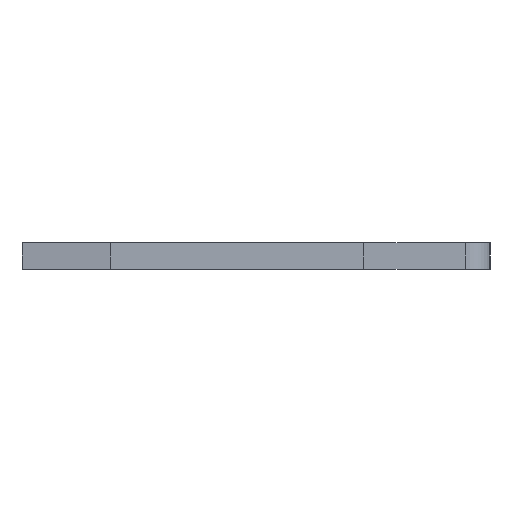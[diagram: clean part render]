
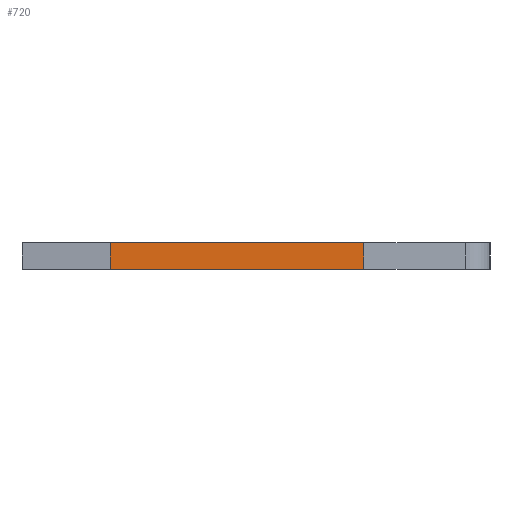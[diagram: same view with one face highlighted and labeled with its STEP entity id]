
A CAD part, left-side view. The second image highlights one B-rep face of the part: STEP entity #720.
In plain terms, the highlighted face is planar.
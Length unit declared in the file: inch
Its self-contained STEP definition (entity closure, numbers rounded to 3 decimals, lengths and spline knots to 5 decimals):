
#8 = ORIENTED_EDGE ( 'NONE', *, *, #1028, .F. ) ;
#26 = DIRECTION ( 'NONE',  ( 1., 0., 0. ) ) ;
#60 = FACE_OUTER_BOUND ( 'NONE', #442, .T. ) ;
#75 = EDGE_CURVE ( 'NONE', #562, #456, #328, .T. ) ;
#207 = CARTESIAN_POINT ( 'NONE',  ( 0.013, 0.146, -0.0575 ) ) ;
#225 = DIRECTION ( 'NONE',  ( -1., 0., 0. ) ) ;
#252 = CARTESIAN_POINT ( 'NONE',  ( 0.013, 0.146, -0.0575 ) ) ;
#278 = ORIENTED_EDGE ( 'NONE', *, *, #1211, .T. ) ;
#295 = ORIENTED_EDGE ( 'NONE', *, *, #411, .F. ) ;
#302 = DIRECTION ( 'NONE',  ( -1., 0., 0. ) ) ;
#310 = VECTOR ( 'NONE', #302, 39.37008 ) ;
#328 = LINE ( 'NONE', #986, #506 ) ;
#332 = VERTEX_POINT ( 'NONE', #1242 ) ;
#375 = DIRECTION ( 'NONE',  ( 0., 0., 1. ) ) ;
#411 = EDGE_CURVE ( 'NONE', #332, #456, #651, .T. ) ;
#414 = DIRECTION ( 'NONE',  ( 0., 1., 0. ) ) ;
#442 = EDGE_LOOP ( 'NONE', ( #1248, #295, #8, #278 ) ) ;
#456 = VERTEX_POINT ( 'NONE', #1024 ) ;
#506 = VECTOR ( 'NONE', #414, 39.37008 ) ;
#562 = VERTEX_POINT ( 'NONE', #906 ) ;
#651 = LINE ( 'NONE', #1144, #1437 ) ;
#720 = ADVANCED_FACE ( 'NONE', ( #60 ), #1267, .F. ) ;
#732 = DIRECTION ( 'NONE',  ( 0., 1., 0. ) ) ;
#906 = CARTESIAN_POINT ( 'NONE',  ( -0.013, -0.099, -0.0575 ) ) ;
#986 = CARTESIAN_POINT ( 'NONE',  ( -0.013, 0.146, -0.0575 ) ) ;
#1024 = CARTESIAN_POINT ( 'NONE',  ( -0.013, 0.146, -0.0575 ) ) ;
#1028 = EDGE_CURVE ( 'NONE', #1309, #332, #1304, .T. ) ;
#1140 = CARTESIAN_POINT ( 'NONE',  ( 0.013, -0.099, -0.0575 ) ) ;
#1144 = CARTESIAN_POINT ( 'NONE',  ( 0.013, 0.146, -0.0575 ) ) ;
#1184 = VECTOR ( 'NONE', #732, 39.37008 ) ;
#1211 = EDGE_CURVE ( 'NONE', #1309, #562, #1423, .T. ) ;
#1242 = CARTESIAN_POINT ( 'NONE',  ( 0.013, 0.146, -0.0575 ) ) ;
#1248 = ORIENTED_EDGE ( 'NONE', *, *, #75, .T. ) ;
#1267 = PLANE ( 'NONE',  #1378 ) ;
#1304 = LINE ( 'NONE', #252, #1184 ) ;
#1309 = VERTEX_POINT ( 'NONE', #1140 ) ;
#1378 = AXIS2_PLACEMENT_3D ( 'NONE', #207, #375, #26 ) ;
#1423 = LINE ( 'NONE', #1464, #310 ) ;
#1437 = VECTOR ( 'NONE', #225, 39.37008 ) ;
#1464 = CARTESIAN_POINT ( 'NONE',  ( 0.013, -0.099, -0.0575 ) ) ;
